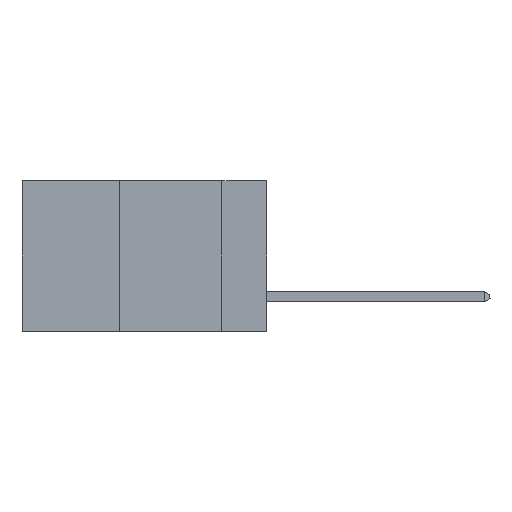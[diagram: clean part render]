
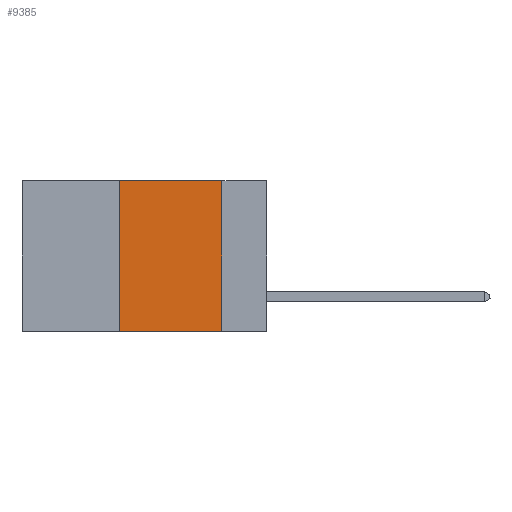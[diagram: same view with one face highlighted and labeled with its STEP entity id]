
A CAD part, left-side view. The second image highlights one B-rep face of the part: STEP entity #9385.
In plain terms, the highlighted planar face has unit normal (-1, 0, 0).
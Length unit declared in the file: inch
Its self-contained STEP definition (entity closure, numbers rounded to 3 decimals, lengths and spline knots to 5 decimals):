
#11 = EDGE_CURVE ( 'NONE', #4158, #326, #17327, .T. ) ;
#326 = VERTEX_POINT ( 'NONE', #5961 ) ;
#1743 = VECTOR ( 'NONE', #25066, 39.37008 ) ;
#1883 = DIRECTION ( 'NONE',  ( 0., 0., -1. ) ) ;
#2472 = DIRECTION ( 'NONE',  ( 1., 0., 0. ) ) ;
#4058 = ORIENTED_EDGE ( 'NONE', *, *, #6195, .F. ) ;
#4158 = VERTEX_POINT ( 'NONE', #9232 ) ;
#4491 = VERTEX_POINT ( 'NONE', #14565 ) ;
#4781 = DIRECTION ( 'NONE',  ( 0., 0., -1. ) ) ;
#4811 = LINE ( 'NONE', #19210, #18419 ) ;
#4838 = VECTOR ( 'NONE', #11822, 39.37008 ) ;
#5792 = CARTESIAN_POINT ( 'NONE',  ( 0., 0.36, 0. ) ) ;
#5961 = CARTESIAN_POINT ( 'NONE',  ( 0., 0.11, -0.37 ) ) ;
#6195 = EDGE_CURVE ( 'NONE', #4158, #22656, #8542, .T. ) ;
#8542 = LINE ( 'NONE', #5792, #4838 ) ;
#8579 = EDGE_CURVE ( 'NONE', #22656, #4491, #10338, .T. ) ;
#9232 = CARTESIAN_POINT ( 'NONE',  ( 0., 0.36, -0.37 ) ) ;
#9385 = ADVANCED_FACE ( 'NONE', ( #13720 ), #14424, .F. ) ;
#10338 = LINE ( 'NONE', #14493, #1743 ) ;
#11822 = DIRECTION ( 'NONE',  ( 0., 0., 1. ) ) ;
#12027 = VECTOR ( 'NONE', #13173, 39.37008 ) ;
#13173 = DIRECTION ( 'NONE',  ( 0., -1., 0. ) ) ;
#13720 = FACE_OUTER_BOUND ( 'NONE', #16178, .T. ) ;
#14424 = PLANE ( 'NONE',  #23472 ) ;
#14493 = CARTESIAN_POINT ( 'NONE',  ( 0., 0.6, 0. ) ) ;
#14565 = CARTESIAN_POINT ( 'NONE',  ( 0., 0.11, 0. ) ) ;
#15430 = ORIENTED_EDGE ( 'NONE', *, *, #24215, .F. ) ;
#15755 = CARTESIAN_POINT ( 'NONE',  ( 0., 0.6, -0.37 ) ) ;
#16178 = EDGE_LOOP ( 'NONE', ( #15430, #16820, #4058, #25083 ) ) ;
#16820 = ORIENTED_EDGE ( 'NONE', *, *, #8579, .F. ) ;
#17327 = LINE ( 'NONE', #15755, #12027 ) ;
#18055 = CARTESIAN_POINT ( 'NONE',  ( 0., 0.36, 0. ) ) ;
#18419 = VECTOR ( 'NONE', #1883, 39.37008 ) ;
#19210 = CARTESIAN_POINT ( 'NONE',  ( 0., 0.11, 0. ) ) ;
#20489 = CARTESIAN_POINT ( 'NONE',  ( 0., 0.6, 0. ) ) ;
#22656 = VERTEX_POINT ( 'NONE', #18055 ) ;
#23472 = AXIS2_PLACEMENT_3D ( 'NONE', #20489, #2472, #4781 ) ;
#24215 = EDGE_CURVE ( 'NONE', #4491, #326, #4811, .T. ) ;
#25066 = DIRECTION ( 'NONE',  ( 0., -1., 0. ) ) ;
#25083 = ORIENTED_EDGE ( 'NONE', *, *, #11, .T. ) ;
